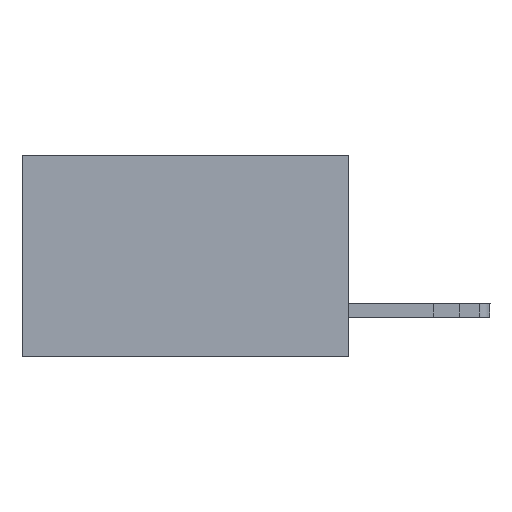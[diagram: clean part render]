
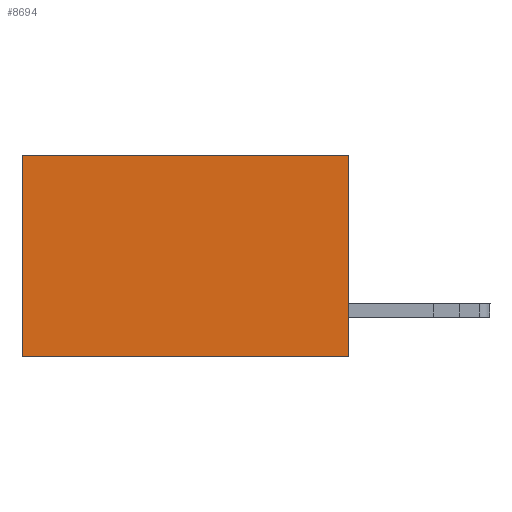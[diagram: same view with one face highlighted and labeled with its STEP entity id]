
A CAD part, left-side view. The second image highlights one B-rep face of the part: STEP entity #8694.
In plain terms, the highlighted planar face has unit normal (-1, 0, 0).
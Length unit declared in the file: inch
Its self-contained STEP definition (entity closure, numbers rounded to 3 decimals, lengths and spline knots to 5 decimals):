
#64 = DIRECTION ( 'NONE',  ( 0., 1., 0. ) ) ;
#913 = CARTESIAN_POINT ( 'NONE',  ( 0.2615, 0., -0.37 ) ) ;
#1483 = CARTESIAN_POINT ( 'NONE',  ( 0.2615, 0.6, -0.37 ) ) ;
#1911 = CARTESIAN_POINT ( 'NONE',  ( 0.2615, 0., -0.37 ) ) ;
#2336 = LINE ( 'NONE', #8512, #7133 ) ;
#2797 = CARTESIAN_POINT ( 'NONE',  ( 0.2615, 0., -0.37 ) ) ;
#2964 = EDGE_LOOP ( 'NONE', ( #14815, #13084, #12309, #5642 ) ) ;
#3180 = LINE ( 'NONE', #4785, #19329 ) ;
#4785 = CARTESIAN_POINT ( 'NONE',  ( 0.2615, 0., 0. ) ) ;
#5642 = ORIENTED_EDGE ( 'NONE', *, *, #13936, .T. ) ;
#5748 = VERTEX_POINT ( 'NONE', #2797 ) ;
#5932 = AXIS2_PLACEMENT_3D ( 'NONE', #913, #11759, #15104 ) ;
#6916 = CARTESIAN_POINT ( 'NONE',  ( 0.2615, 0., 0. ) ) ;
#6988 = FACE_OUTER_BOUND ( 'NONE', #2964, .T. ) ;
#7000 = DIRECTION ( 'NONE',  ( 0., 1., 0. ) ) ;
#7133 = VECTOR ( 'NONE', #7000, 39.37008 ) ;
#7950 = CARTESIAN_POINT ( 'NONE',  ( 0.2615, 0.6, 0. ) ) ;
#8512 = CARTESIAN_POINT ( 'NONE',  ( 0.2615, 0., -0.37 ) ) ;
#8694 = ADVANCED_FACE ( 'NONE', ( #6988 ), #10239, .F. ) ;
#9340 = VERTEX_POINT ( 'NONE', #7950 ) ;
#10239 = PLANE ( 'NONE',  #5932 ) ;
#11227 = LINE ( 'NONE', #1911, #19603 ) ;
#11759 = DIRECTION ( 'NONE',  ( 1., 0., 0. ) ) ;
#11850 = EDGE_CURVE ( 'NONE', #14322, #5748, #11227, .T. ) ;
#12309 = ORIENTED_EDGE ( 'NONE', *, *, #11850, .F. ) ;
#12893 = CARTESIAN_POINT ( 'NONE',  ( 0.2615, 0.6, -0.37 ) ) ;
#13084 = ORIENTED_EDGE ( 'NONE', *, *, #17359, .F. ) ;
#13936 = EDGE_CURVE ( 'NONE', #14322, #9340, #3180, .T. ) ;
#14322 = VERTEX_POINT ( 'NONE', #6916 ) ;
#14815 = ORIENTED_EDGE ( 'NONE', *, *, #18839, .T. ) ;
#15104 = DIRECTION ( 'NONE',  ( 0., 0., -1. ) ) ;
#15731 = LINE ( 'NONE', #1483, #16910 ) ;
#15864 = VERTEX_POINT ( 'NONE', #12893 ) ;
#16910 = VECTOR ( 'NONE', #17161, 39.37008 ) ;
#17161 = DIRECTION ( 'NONE',  ( 0., 0., -1. ) ) ;
#17359 = EDGE_CURVE ( 'NONE', #5748, #15864, #2336, .T. ) ;
#17628 = DIRECTION ( 'NONE',  ( 0., 0., -1. ) ) ;
#18839 = EDGE_CURVE ( 'NONE', #9340, #15864, #15731, .T. ) ;
#19329 = VECTOR ( 'NONE', #64, 39.37008 ) ;
#19603 = VECTOR ( 'NONE', #17628, 39.37008 ) ;
